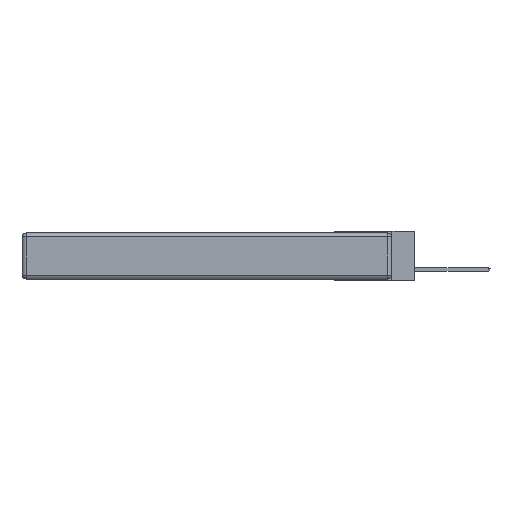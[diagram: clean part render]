
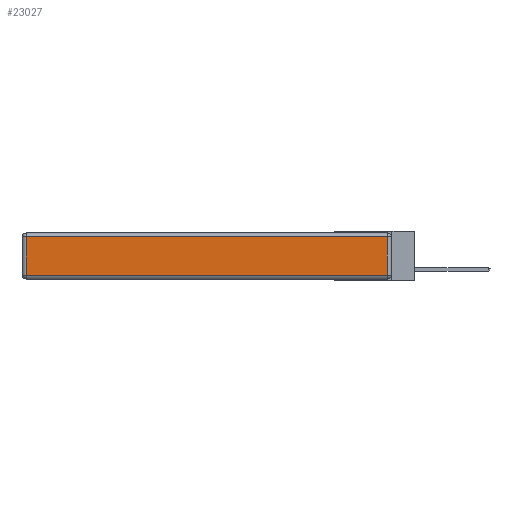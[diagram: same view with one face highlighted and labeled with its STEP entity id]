
A CAD part, left-side view. The second image highlights one B-rep face of the part: STEP entity #23027.
In plain terms, the highlighted planar face has unit normal (-1, 0, 0).
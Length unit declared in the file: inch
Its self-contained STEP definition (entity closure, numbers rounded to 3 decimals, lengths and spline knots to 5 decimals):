
#323 = ORIENTED_EDGE ( 'NONE', *, *, #21169, .T. ) ;
#769 = VERTEX_POINT ( 'NONE', #19472 ) ;
#816 = ORIENTED_EDGE ( 'NONE', *, *, #11422, .T. ) ;
#927 = CARTESIAN_POINT ( 'NONE',  ( 0., 2.72, -0.343 ) ) ;
#1768 = DIRECTION ( 'NONE',  ( 0., -1., 0. ) ) ;
#2062 = EDGE_CURVE ( 'NONE', #15942, #769, #15305, .T. ) ;
#2280 = VECTOR ( 'NONE', #14539, 39.37008 ) ;
#2955 = DIRECTION ( 'NONE',  ( 0., 1., 0. ) ) ;
#3173 = VERTEX_POINT ( 'NONE', #18680 ) ;
#3288 = VECTOR ( 'NONE', #3480, 39.37008 ) ;
#3346 = EDGE_CURVE ( 'NONE', #3173, #18896, #24491, .T. ) ;
#3480 = DIRECTION ( 'NONE',  ( 0., 0., 1. ) ) ;
#7338 = ORIENTED_EDGE ( 'NONE', *, *, #2062, .T. ) ;
#8312 = ORIENTED_EDGE ( 'NONE', *, *, #3346, .T. ) ;
#8343 = DIRECTION ( 'NONE',  ( -1., 0., 0. ) ) ;
#9468 = FACE_OUTER_BOUND ( 'NONE', #19682, .T. ) ;
#9565 = CARTESIAN_POINT ( 'NONE',  ( 0., 0.03, -0.343 ) ) ;
#10252 = VECTOR ( 'NONE', #1768, 39.37008 ) ;
#11422 = EDGE_CURVE ( 'NONE', #769, #3173, #20705, .T. ) ;
#11643 = CARTESIAN_POINT ( 'NONE',  ( 0., 0., -0.313 ) ) ;
#14539 = DIRECTION ( 'NONE',  ( 0., 0., -1. ) ) ;
#15305 = LINE ( 'NONE', #11643, #10252 ) ;
#15942 = VERTEX_POINT ( 'NONE', #23306 ) ;
#17849 = PLANE ( 'NONE',  #23476 ) ;
#18680 = CARTESIAN_POINT ( 'NONE',  ( 0., 0.03, -0.03 ) ) ;
#18896 = VERTEX_POINT ( 'NONE', #22084 ) ;
#19472 = CARTESIAN_POINT ( 'NONE',  ( 0., 0.03, -0.313 ) ) ;
#19682 = EDGE_LOOP ( 'NONE', ( #7338, #816, #8312, #323 ) ) ;
#19770 = CARTESIAN_POINT ( 'NONE',  ( 0., 0., -0.343 ) ) ;
#19892 = CARTESIAN_POINT ( 'NONE',  ( 0., 2.75, -0.03 ) ) ;
#20705 = LINE ( 'NONE', #9565, #3288 ) ;
#21169 = EDGE_CURVE ( 'NONE', #18896, #15942, #22365, .T. ) ;
#21715 = DIRECTION ( 'NONE',  ( 0., 0., 1. ) ) ;
#22084 = CARTESIAN_POINT ( 'NONE',  ( 0., 2.72, -0.03 ) ) ;
#22365 = LINE ( 'NONE', #927, #2280 ) ;
#23027 = ADVANCED_FACE ( 'NONE', ( #9468 ), #17849, .T. ) ;
#23306 = CARTESIAN_POINT ( 'NONE',  ( 0., 2.72, -0.313 ) ) ;
#23476 = AXIS2_PLACEMENT_3D ( 'NONE', #19770, #8343, #21715 ) ;
#24491 = LINE ( 'NONE', #19892, #24781 ) ;
#24781 = VECTOR ( 'NONE', #2955, 39.37008 ) ;
